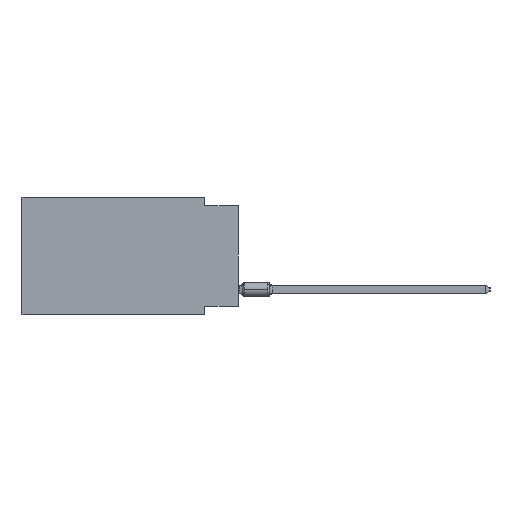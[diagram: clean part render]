
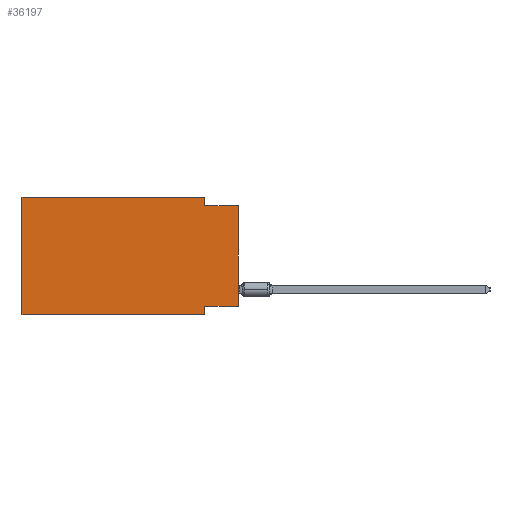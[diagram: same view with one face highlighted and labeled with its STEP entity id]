
A CAD part, left-side view. The second image highlights one B-rep face of the part: STEP entity #36197.
In plain terms, the highlighted planar face has unit normal (-1, 0, 0).
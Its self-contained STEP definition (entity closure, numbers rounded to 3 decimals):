
#2062 = LINE ( 'NONE', #26295, #16368 ) ;
#2289 = EDGE_LOOP ( 'NONE', ( #38170, #44226, #6832, #24711, #16282, #38971, #41559, #38782 ) ) ;
#2417 = DIRECTION ( 'NONE',  ( 0., -1., 0. ) ) ;
#2971 = CARTESIAN_POINT ( 'NONE',  ( 0., 0., 0. ) ) ;
#3107 = CARTESIAN_POINT ( 'NONE',  ( 0., 2.54, 0. ) ) ;
#3183 = CARTESIAN_POINT ( 'NONE',  ( 0., 16.383, 0. ) ) ;
#4793 = VECTOR ( 'NONE', #5101, 1000. ) ;
#5101 = DIRECTION ( 'NONE',  ( 0., 0., -1. ) ) ;
#6212 = CARTESIAN_POINT ( 'NONE',  ( 0., 16.383, 0. ) ) ;
#6832 = ORIENTED_EDGE ( 'NONE', *, *, #43510, .F. ) ;
#8858 = LINE ( 'NONE', #9090, #9213 ) ;
#9000 = CARTESIAN_POINT ( 'NONE',  ( 0., 0., -0.635 ) ) ;
#9003 = VECTOR ( 'NONE', #9203, 1000. ) ;
#9090 = CARTESIAN_POINT ( 'NONE',  ( 0., 0., -0.635 ) ) ;
#9165 = LINE ( 'NONE', #22867, #33771 ) ;
#9203 = DIRECTION ( 'NONE',  ( 0., 0., -1. ) ) ;
#9213 = VECTOR ( 'NONE', #40275, 1000. ) ;
#11557 = DIRECTION ( 'NONE',  ( 0., 0., 1. ) ) ;
#12673 = EDGE_CURVE ( 'NONE', #13949, #27418, #9165, .T. ) ;
#13006 = LINE ( 'NONE', #30506, #9003 ) ;
#13949 = VERTEX_POINT ( 'NONE', #34858 ) ;
#14064 = CARTESIAN_POINT ( 'NONE',  ( 0., 0., -8.255 ) ) ;
#14234 = CARTESIAN_POINT ( 'NONE',  ( 0., 2.54, -0.635 ) ) ;
#16282 = ORIENTED_EDGE ( 'NONE', *, *, #22938, .F. ) ;
#16368 = VECTOR ( 'NONE', #29881, 1000. ) ;
#16749 = LINE ( 'NONE', #6212, #32793 ) ;
#17749 = VERTEX_POINT ( 'NONE', #9000 ) ;
#18578 = CARTESIAN_POINT ( 'NONE',  ( 0., 16.383, 0. ) ) ;
#21605 = AXIS2_PLACEMENT_3D ( 'NONE', #3183, #30342, #33950 ) ;
#21718 = LINE ( 'NONE', #42596, #4793 ) ;
#22124 = VECTOR ( 'NONE', #11557, 1000. ) ;
#22867 = CARTESIAN_POINT ( 'NONE',  ( 0., 16.383, -8.89 ) ) ;
#22938 = EDGE_CURVE ( 'NONE', #13949, #24285, #42324, .T. ) ;
#23622 = FACE_OUTER_BOUND ( 'NONE', #2289, .T. ) ;
#24157 = EDGE_CURVE ( 'NONE', #25288, #27418, #21718, .T. ) ;
#24285 = VERTEX_POINT ( 'NONE', #18578 ) ;
#24711 = ORIENTED_EDGE ( 'NONE', *, *, #33857, .F. ) ;
#25288 = VERTEX_POINT ( 'NONE', #33667 ) ;
#25958 = EDGE_CURVE ( 'NONE', #38814, #17749, #8858, .T. ) ;
#26295 = CARTESIAN_POINT ( 'NONE',  ( 0., 0., -8.255 ) ) ;
#27418 = VERTEX_POINT ( 'NONE', #38219 ) ;
#28654 = DIRECTION ( 'NONE',  ( 0., -1., 0. ) ) ;
#29285 = CARTESIAN_POINT ( 'NONE',  ( 0., 16.383, 0. ) ) ;
#29881 = DIRECTION ( 'NONE',  ( 0., 1., 0. ) ) ;
#30342 = DIRECTION ( 'NONE',  ( 1., 0., 0. ) ) ;
#30506 = CARTESIAN_POINT ( 'NONE',  ( 0., 2.54, 0. ) ) ;
#30810 = VECTOR ( 'NONE', #36220, 1000. ) ;
#32793 = VECTOR ( 'NONE', #28654, 1000. ) ;
#33667 = CARTESIAN_POINT ( 'NONE',  ( 0., 2.54, -8.255 ) ) ;
#33771 = VECTOR ( 'NONE', #2417, 1000. ) ;
#33857 = EDGE_CURVE ( 'NONE', #24285, #42470, #16749, .T. ) ;
#33950 = DIRECTION ( 'NONE',  ( 0., 0., -1. ) ) ;
#34241 = EDGE_CURVE ( 'NONE', #42220, #25288, #2062, .T. ) ;
#34858 = CARTESIAN_POINT ( 'NONE',  ( 0., 16.383, -8.89 ) ) ;
#36197 = ADVANCED_FACE ( 'NONE', ( #23622 ), #37316, .F. ) ;
#36220 = DIRECTION ( 'NONE',  ( 0., 0., 1. ) ) ;
#37316 = PLANE ( 'NONE',  #21605 ) ;
#38170 = ORIENTED_EDGE ( 'NONE', *, *, #41372, .T. ) ;
#38219 = CARTESIAN_POINT ( 'NONE',  ( 0., 2.54, -8.89 ) ) ;
#38782 = ORIENTED_EDGE ( 'NONE', *, *, #34241, .F. ) ;
#38814 = VERTEX_POINT ( 'NONE', #14234 ) ;
#38971 = ORIENTED_EDGE ( 'NONE', *, *, #12673, .T. ) ;
#40275 = DIRECTION ( 'NONE',  ( 0., -1., 0. ) ) ;
#41372 = EDGE_CURVE ( 'NONE', #42220, #17749, #43178, .T. ) ;
#41559 = ORIENTED_EDGE ( 'NONE', *, *, #24157, .F. ) ;
#42220 = VERTEX_POINT ( 'NONE', #14064 ) ;
#42324 = LINE ( 'NONE', #29285, #22124 ) ;
#42470 = VERTEX_POINT ( 'NONE', #3107 ) ;
#42596 = CARTESIAN_POINT ( 'NONE',  ( 0., 2.54, -8.89 ) ) ;
#43178 = LINE ( 'NONE', #2971, #30810 ) ;
#43510 = EDGE_CURVE ( 'NONE', #42470, #38814, #13006, .T. ) ;
#44226 = ORIENTED_EDGE ( 'NONE', *, *, #25958, .F. ) ;
